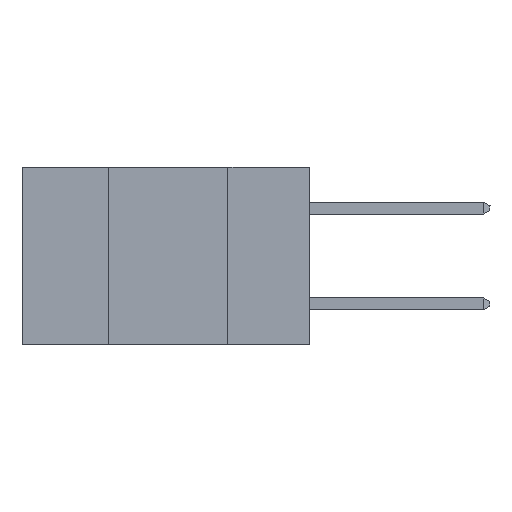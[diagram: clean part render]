
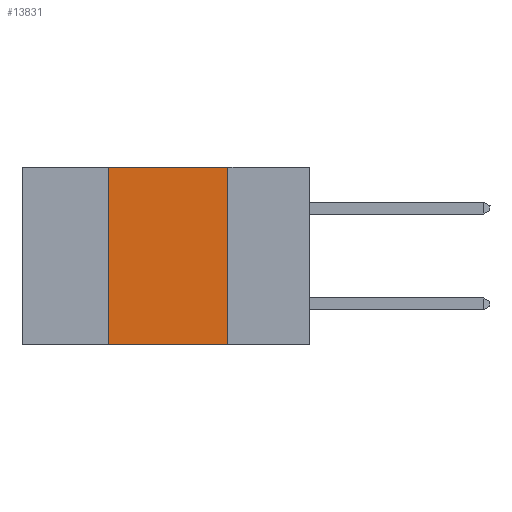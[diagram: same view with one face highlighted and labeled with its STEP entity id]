
A CAD part, left-side view. The second image highlights one B-rep face of the part: STEP entity #13831.
In plain terms, the highlighted planar face has unit normal (-1, 0, 0).
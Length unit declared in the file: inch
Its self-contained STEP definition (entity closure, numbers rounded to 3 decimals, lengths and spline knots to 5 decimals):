
#202 = PLANE ( 'NONE',  #27406 ) ;
#406 = VECTOR ( 'NONE', #17548, 39.37008 ) ;
#1201 = CARTESIAN_POINT ( 'NONE',  ( 0., 0.17, 0. ) ) ;
#1467 = CARTESIAN_POINT ( 'NONE',  ( 0., 0.42, 0. ) ) ;
#2898 = LINE ( 'NONE', #1467, #406 ) ;
#2997 = ORIENTED_EDGE ( 'NONE', *, *, #15706, .F. ) ;
#3485 = DIRECTION ( 'NONE',  ( 0., 0., -1. ) ) ;
#5248 = ORIENTED_EDGE ( 'NONE', *, *, #22045, .F. ) ;
#5300 = CARTESIAN_POINT ( 'NONE',  ( 0., 0.42, 0. ) ) ;
#6816 = VERTEX_POINT ( 'NONE', #20889 ) ;
#7108 = CARTESIAN_POINT ( 'NONE',  ( 0., 0.6, 0. ) ) ;
#7575 = VERTEX_POINT ( 'NONE', #14383 ) ;
#8230 = ORIENTED_EDGE ( 'NONE', *, *, #10691, .F. ) ;
#9155 = EDGE_LOOP ( 'NONE', ( #2997, #5248, #8230, #10215 ) ) ;
#9342 = CARTESIAN_POINT ( 'NONE',  ( 0., 0.6, -0.37 ) ) ;
#9414 = DIRECTION ( 'NONE',  ( 0., 0., -1. ) ) ;
#9667 = VECTOR ( 'NONE', #3485, 39.37008 ) ;
#10215 = ORIENTED_EDGE ( 'NONE', *, *, #17428, .T. ) ;
#10411 = LINE ( 'NONE', #1201, #9667 ) ;
#10691 = EDGE_CURVE ( 'NONE', #6816, #15225, #2898, .T. ) ;
#11103 = LINE ( 'NONE', #20660, #22646 ) ;
#11739 = VECTOR ( 'NONE', #23162, 39.37008 ) ;
#12588 = VERTEX_POINT ( 'NONE', #19056 ) ;
#12781 = FACE_OUTER_BOUND ( 'NONE', #9155, .T. ) ;
#13831 = ADVANCED_FACE ( 'NONE', ( #12781 ), #202, .F. ) ;
#14383 = CARTESIAN_POINT ( 'NONE',  ( 0., 0.17, 0. ) ) ;
#15225 = VERTEX_POINT ( 'NONE', #5300 ) ;
#15706 = EDGE_CURVE ( 'NONE', #7575, #12588, #10411, .T. ) ;
#17428 = EDGE_CURVE ( 'NONE', #6816, #12588, #17863, .T. ) ;
#17548 = DIRECTION ( 'NONE',  ( 0., 0., 1. ) ) ;
#17863 = LINE ( 'NONE', #9342, #11739 ) ;
#19056 = CARTESIAN_POINT ( 'NONE',  ( 0., 0.17, -0.37 ) ) ;
#20660 = CARTESIAN_POINT ( 'NONE',  ( 0., 0.6, 0. ) ) ;
#20889 = CARTESIAN_POINT ( 'NONE',  ( 0., 0.42, -0.37 ) ) ;
#22045 = EDGE_CURVE ( 'NONE', #15225, #7575, #11103, .T. ) ;
#22646 = VECTOR ( 'NONE', #23009, 39.37008 ) ;
#23009 = DIRECTION ( 'NONE',  ( 0., -1., 0. ) ) ;
#23162 = DIRECTION ( 'NONE',  ( 0., -1., 0. ) ) ;
#23259 = DIRECTION ( 'NONE',  ( 1., 0., 0. ) ) ;
#27406 = AXIS2_PLACEMENT_3D ( 'NONE', #7108, #23259, #9414 ) ;
